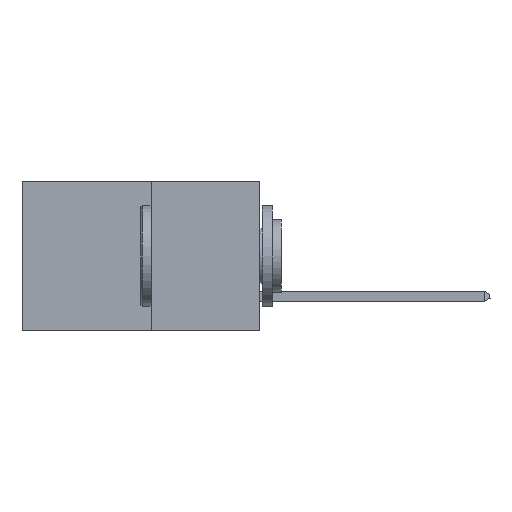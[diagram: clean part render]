
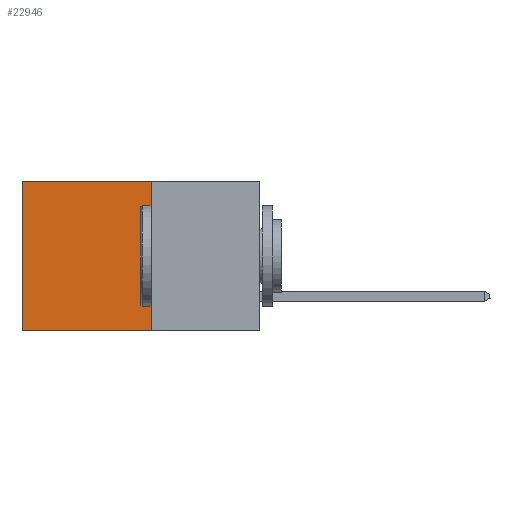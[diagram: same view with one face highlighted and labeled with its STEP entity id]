
A CAD part, left-side view. The second image highlights one B-rep face of the part: STEP entity #22946.
In plain terms, the highlighted planar face has unit normal (-1, 0, 0).
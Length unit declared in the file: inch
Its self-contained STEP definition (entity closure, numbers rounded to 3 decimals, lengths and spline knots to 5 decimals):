
#236 = FACE_OUTER_BOUND ( 'NONE', #11175, .T. ) ;
#341 = VERTEX_POINT ( 'NONE', #4276 ) ;
#646 = EDGE_CURVE ( 'NONE', #341, #27302, #4320, .T. ) ;
#2442 = DIRECTION ( 'NONE',  ( 0., 1., 0. ) ) ;
#2831 = CARTESIAN_POINT ( 'NONE',  ( 0.277, 0.59, -0.37 ) ) ;
#4276 = CARTESIAN_POINT ( 'NONE',  ( 0.277, 0.27, -0.37 ) ) ;
#4320 = LINE ( 'NONE', #8614, #29817 ) ;
#5269 = EDGE_CURVE ( 'NONE', #8772, #341, #30280, .T. ) ;
#5914 = VERTEX_POINT ( 'NONE', #27862 ) ;
#6332 = CARTESIAN_POINT ( 'NONE',  ( 0.277, 0.27, 0. ) ) ;
#7721 = DIRECTION ( 'NONE',  ( 0., 0., -1. ) ) ;
#8461 = DIRECTION ( 'NONE',  ( 0., 1., 0. ) ) ;
#8614 = CARTESIAN_POINT ( 'NONE',  ( 0.277, 0.27, -0.37 ) ) ;
#8772 = VERTEX_POINT ( 'NONE', #6332 ) ;
#9865 = CARTESIAN_POINT ( 'NONE',  ( 0.277, 0.59, -0.37 ) ) ;
#10012 = ORIENTED_EDGE ( 'NONE', *, *, #21390, .T. ) ;
#11175 = EDGE_LOOP ( 'NONE', ( #18688, #19213, #17136, #10012 ) ) ;
#11434 = CARTESIAN_POINT ( 'NONE',  ( 0.277, 0.27, -0.37 ) ) ;
#12297 = CARTESIAN_POINT ( 'NONE',  ( 0.277, 0.27, 0. ) ) ;
#13918 = LINE ( 'NONE', #2831, #18873 ) ;
#13961 = DIRECTION ( 'NONE',  ( 0., 0., -1. ) ) ;
#16383 = VECTOR ( 'NONE', #26432, 39.37008 ) ;
#17136 = ORIENTED_EDGE ( 'NONE', *, *, #5269, .F. ) ;
#18688 = ORIENTED_EDGE ( 'NONE', *, *, #27407, .T. ) ;
#18873 = VECTOR ( 'NONE', #7721, 39.37008 ) ;
#19213 = ORIENTED_EDGE ( 'NONE', *, *, #646, .F. ) ;
#21390 = EDGE_CURVE ( 'NONE', #8772, #5914, #28569, .T. ) ;
#21999 = VECTOR ( 'NONE', #2442, 39.37008 ) ;
#22038 = AXIS2_PLACEMENT_3D ( 'NONE', #11434, #28698, #13961 ) ;
#22946 = ADVANCED_FACE ( 'NONE', ( #236 ), #23725, .F. ) ;
#23725 = PLANE ( 'NONE',  #22038 ) ;
#26221 = CARTESIAN_POINT ( 'NONE',  ( 0.277, 0.27, -0.37 ) ) ;
#26432 = DIRECTION ( 'NONE',  ( 0., 0., -1. ) ) ;
#27302 = VERTEX_POINT ( 'NONE', #9865 ) ;
#27407 = EDGE_CURVE ( 'NONE', #5914, #27302, #13918, .T. ) ;
#27862 = CARTESIAN_POINT ( 'NONE',  ( 0.277, 0.59, 0. ) ) ;
#28569 = LINE ( 'NONE', #12297, #21999 ) ;
#28698 = DIRECTION ( 'NONE',  ( 1., 0., 0. ) ) ;
#29817 = VECTOR ( 'NONE', #8461, 39.37008 ) ;
#30280 = LINE ( 'NONE', #26221, #16383 ) ;
